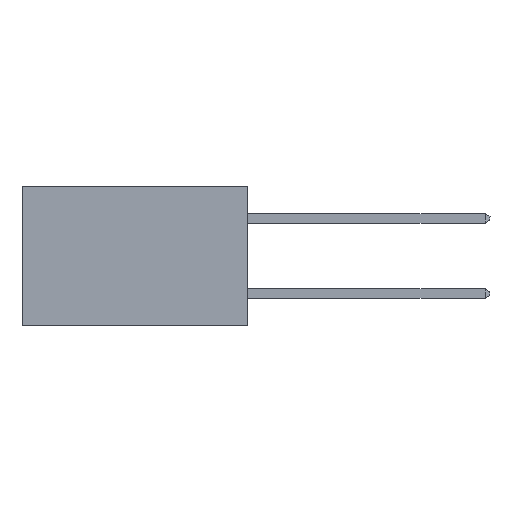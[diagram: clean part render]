
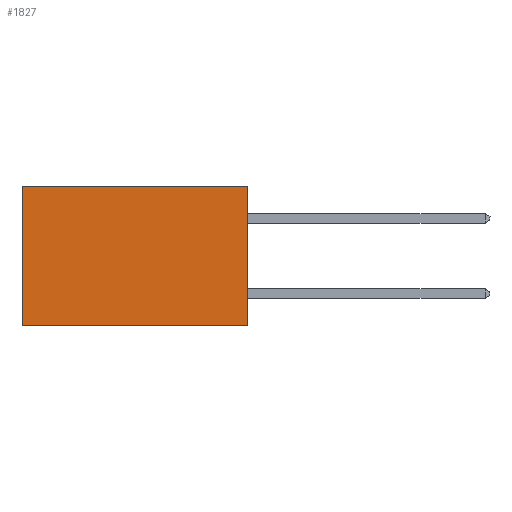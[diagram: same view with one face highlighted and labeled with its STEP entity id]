
A CAD part, left-side view. The second image highlights one B-rep face of the part: STEP entity #1827.
In plain terms, the highlighted planar face has unit normal (-1, 0, 0).
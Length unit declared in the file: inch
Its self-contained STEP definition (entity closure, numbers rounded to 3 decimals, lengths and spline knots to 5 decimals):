
#69 = LINE ( 'NONE', #9551, #8155 ) ;
#471 = ORIENTED_EDGE ( 'NONE', *, *, #6033, .F. ) ;
#555 = EDGE_CURVE ( 'NONE', #4583, #1192, #9606, .T. ) ;
#645 = DIRECTION ( 'NONE',  ( 0., 1., 0. ) ) ;
#1192 = VERTEX_POINT ( 'NONE', #1930 ) ;
#1358 = CARTESIAN_POINT ( 'NONE',  ( 0.2615, 0., 0. ) ) ;
#1388 = LINE ( 'NONE', #3012, #2594 ) ;
#1669 = DIRECTION ( 'NONE',  ( 0., 1., 0. ) ) ;
#1827 = ADVANCED_FACE ( 'NONE', ( #4875 ), #5873, .F. ) ;
#1930 = CARTESIAN_POINT ( 'NONE',  ( 0.2615, 0.6, -0.37 ) ) ;
#2221 = DIRECTION ( 'NONE',  ( 0., 0., -1. ) ) ;
#2428 = EDGE_CURVE ( 'NONE', #5094, #8992, #1388, .T. ) ;
#2594 = VECTOR ( 'NONE', #2221, 39.37008 ) ;
#2742 = CARTESIAN_POINT ( 'NONE',  ( 0.2615, 0.6, 0. ) ) ;
#3012 = CARTESIAN_POINT ( 'NONE',  ( 0.2615, 0., -0.37 ) ) ;
#3620 = DIRECTION ( 'NONE',  ( 0., 0., -1. ) ) ;
#3781 = AXIS2_PLACEMENT_3D ( 'NONE', #5885, #8343, #3620 ) ;
#4044 = VECTOR ( 'NONE', #645, 39.37008 ) ;
#4184 = CARTESIAN_POINT ( 'NONE',  ( 0.2615, 0.6, -0.37 ) ) ;
#4583 = VERTEX_POINT ( 'NONE', #2742 ) ;
#4799 = EDGE_CURVE ( 'NONE', #5094, #4583, #69, .T. ) ;
#4875 = FACE_OUTER_BOUND ( 'NONE', #9729, .T. ) ;
#5094 = VERTEX_POINT ( 'NONE', #1358 ) ;
#5789 = ORIENTED_EDGE ( 'NONE', *, *, #555, .T. ) ;
#5873 = PLANE ( 'NONE',  #3781 ) ;
#5885 = CARTESIAN_POINT ( 'NONE',  ( 0.2615, 0., -0.37 ) ) ;
#6033 = EDGE_CURVE ( 'NONE', #8992, #1192, #7815, .T. ) ;
#6178 = CARTESIAN_POINT ( 'NONE',  ( 0.2615, 0., -0.37 ) ) ;
#7476 = ORIENTED_EDGE ( 'NONE', *, *, #2428, .F. ) ;
#7815 = LINE ( 'NONE', #8810, #4044 ) ;
#8092 = DIRECTION ( 'NONE',  ( 0., 0., -1. ) ) ;
#8155 = VECTOR ( 'NONE', #1669, 39.37008 ) ;
#8343 = DIRECTION ( 'NONE',  ( 1., 0., 0. ) ) ;
#8810 = CARTESIAN_POINT ( 'NONE',  ( 0.2615, 0., -0.37 ) ) ;
#8992 = VERTEX_POINT ( 'NONE', #6178 ) ;
#9289 = VECTOR ( 'NONE', #8092, 39.37008 ) ;
#9544 = ORIENTED_EDGE ( 'NONE', *, *, #4799, .T. ) ;
#9551 = CARTESIAN_POINT ( 'NONE',  ( 0.2615, 0., 0. ) ) ;
#9606 = LINE ( 'NONE', #4184, #9289 ) ;
#9729 = EDGE_LOOP ( 'NONE', ( #5789, #471, #7476, #9544 ) ) ;
